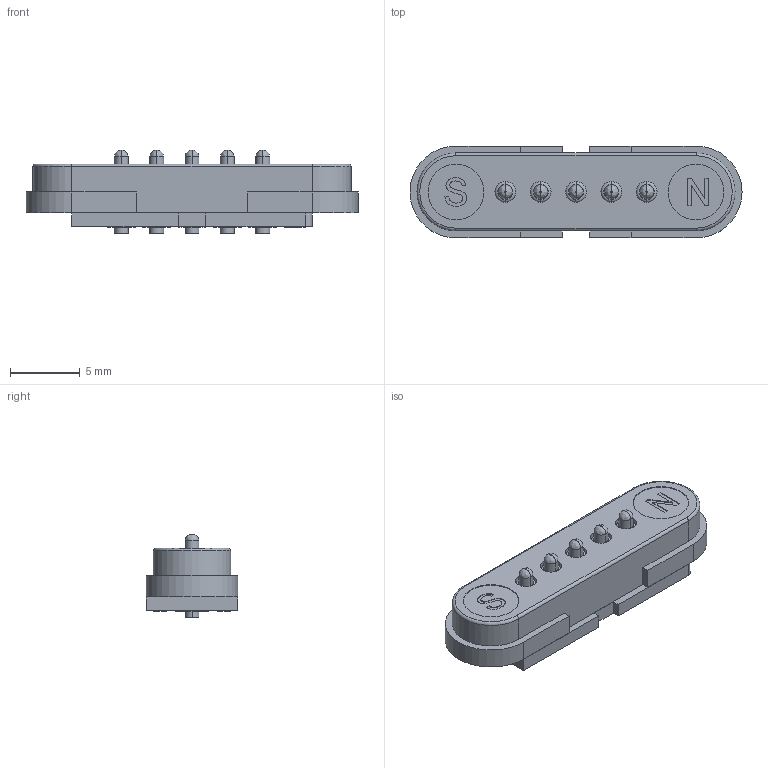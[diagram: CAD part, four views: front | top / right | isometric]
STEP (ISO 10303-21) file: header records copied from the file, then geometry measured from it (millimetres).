
FILE_DESCRIPTION (( 'STEP AP203' ), '1' );
FILE_NAME ('685-D05C2P51110.STEP', '2023-02-07T12:29:10', ( '' ), ( '' ), 'SwSTEP 2.0', 'SolidWorks 2020', '' );
FILE_SCHEMA (( 'CONFIG_CONTROL_DESIGN' ));
Length unit declared in the file: millimetre
Products named in the file (1): 685-D05C2P51110
Bounding box: 23.86 x 6.6 x 6 mm (x, y, z)
Volume: 529.4 mm3; surface area: 976.2 mm2
Topology: 11 solids, 11 shells, 244 faces, 563 edges, 354 vertices
Faces by surface type: plane 107, cylinder 87, bspline 24, torus 16, cone 10
Entity records: 7976 total; most frequent: CARTESIAN_POINT 2332, DIRECTION 1199, ORIENTED_EDGE 1106, EDGE_CURVE 553, AXIS2_PLACEMENT_3D 453, VERTEX_POINT 354, LINE 293, VECTOR 293
